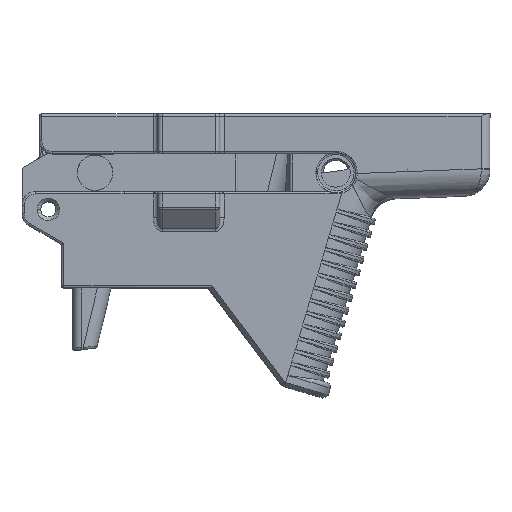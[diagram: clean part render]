
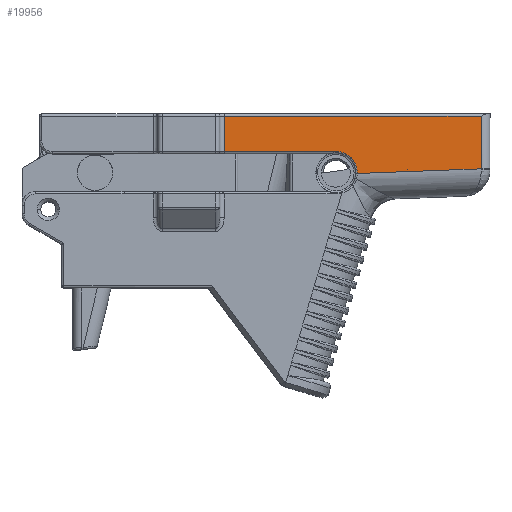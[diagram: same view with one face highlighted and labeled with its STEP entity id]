
A CAD part, top view. The second image highlights one B-rep face of the part: STEP entity #19956.
In plain terms, the highlighted planar face has unit normal (0, 0, 1).
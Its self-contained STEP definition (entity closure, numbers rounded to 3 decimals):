
#33 = LINE ( 'NONE', #19296, #10130 ) ;
#641 = CARTESIAN_POINT ( 'NONE',  ( -48.401, -16.834, 20. ) ) ;
#1420 = CARTESIAN_POINT ( 'NONE',  ( -19.732, -18.269, 20. ) ) ;
#1574 = CARTESIAN_POINT ( 'NONE',  ( -18.826, -19.573, 20. ) ) ;
#1768 = LINE ( 'NONE', #29862, #4794 ) ;
#1918 = EDGE_CURVE ( 'NONE', #3458, #27652, #27993, .T. ) ;
#1987 = VECTOR ( 'NONE', #25201, 1000. ) ;
#2001 = DIRECTION ( 'NONE',  ( 1., 0., 0. ) ) ;
#2130 = CARTESIAN_POINT ( 'NONE',  ( -22.304, -16.888, 20. ) ) ;
#2951 = LINE ( 'NONE', #641, #16053 ) ;
#3097 = CARTESIAN_POINT ( 'NONE',  ( -19.732, -18.269, 20. ) ) ;
#3452 = CARTESIAN_POINT ( 'NONE',  ( -7.079, -20.83, 20. ) ) ;
#3458 = VERTEX_POINT ( 'NONE', #3097 ) ;
#3650 = LINE ( 'NONE', #24642, #8171 ) ;
#3836 = CARTESIAN_POINT ( 'NONE',  ( -22.772, -16.821, 20. ) ) ;
#3881 = CARTESIAN_POINT ( 'NONE',  ( -19.232, -18.88, 20. ) ) ;
#4056 = CARTESIAN_POINT ( 'NONE',  ( -23.365, -16.81, 20. ) ) ;
#4072 = VERTEX_POINT ( 'NONE', #4056 ) ;
#4141 = CARTESIAN_POINT ( 'NONE',  ( -23.167, -16.81, 20. ) ) ;
#4289 = CARTESIAN_POINT ( 'NONE',  ( -21.907, -16.967, 20. ) ) ;
#4794 = VECTOR ( 'NONE', #6690, 1000. ) ;
#4997 = EDGE_CURVE ( 'NONE', #20384, #25131, #26911, .T. ) ;
#5338 = LINE ( 'NONE', #9688, #8516 ) ;
#5424 = EDGE_CURVE ( 'NONE', #12970, #10039, #16466, .T. ) ;
#5905 = CARTESIAN_POINT ( 'NONE',  ( -19.622, -18.383, 20. ) ) ;
#5996 = DIRECTION ( 'NONE',  ( 0., 0., 1. ) ) ;
#6203 = CARTESIAN_POINT ( 'NONE',  ( -19.324, -18.751, 20. ) ) ;
#6354 = CARTESIAN_POINT ( 'NONE',  ( -18.485, -20.649, 20. ) ) ;
#6442 = VECTOR ( 'NONE', #19225, 1000. ) ;
#6464 = CARTESIAN_POINT ( 'NONE',  ( -22.537, -16.851, 20. ) ) ;
#6690 = DIRECTION ( 'NONE',  ( -0.999, -0.037, 0. ) ) ;
#7257 = ORIENTED_EDGE ( 'NONE', *, *, #5424, .F. ) ;
#8138 = DIRECTION ( 'NONE',  ( 0., -1., 0. ) ) ;
#8170 = LINE ( 'NONE', #14798, #9673 ) ;
#8171 = VECTOR ( 'NONE', #8138, 1000. ) ;
#8516 = VECTOR ( 'NONE', #19075, 1000. ) ;
#8923 = B_SPLINE_CURVE_WITH_KNOTS ( 'NONE', 3,
 ( #4141, #22808, #3836, #6464, #16027, #2130, #4289, #20498, #23257, #23104, #25134, #11248, #22955, #27618, #9090, #25284 ),
 .UNSPECIFIED., .F., .F.,
 ( 4, 1, 2, 2, 2, 1, 2, 2, 4 ),
 ( 0., 0.063, 0.094, 0.125, 0.25, 0.313, 0.344, 0.375, 0.5 ),
 .UNSPECIFIED. ) ;
#9090 = CARTESIAN_POINT ( 'NONE',  ( -19.952, -18.041, 20. ) ) ;
#9254 = CARTESIAN_POINT ( 'NONE',  ( -76.723, -16.81, 20. ) ) ;
#9367 = CARTESIAN_POINT ( 'NONE',  ( -48.401, -8.822, 20. ) ) ;
#9673 = VECTOR ( 'NONE', #17415, 1000. ) ;
#9688 = CARTESIAN_POINT ( 'NONE',  ( 9.532, -32.155, 20. ) ) ;
#10039 = VERTEX_POINT ( 'NONE', #11612 ) ;
#10130 = VECTOR ( 'NONE', #19145, 1000. ) ;
#10252 = ORIENTED_EDGE ( 'NONE', *, *, #11085, .F. ) ;
#10475 = PLANE ( 'NONE',  #20900 ) ;
#10712 = VERTEX_POINT ( 'NONE', #14435 ) ;
#10947 = CARTESIAN_POINT ( 'NONE',  ( -18.397, -21.754, 20. ) ) ;
#11039 = VECTOR ( 'NONE', #2001, 1000. ) ;
#11085 = EDGE_CURVE ( 'NONE', #12878, #27652, #1768, .T. ) ;
#11136 = CARTESIAN_POINT ( 'NONE',  ( -18.386, -21.436, 20. ) ) ;
#11248 = CARTESIAN_POINT ( 'NONE',  ( -20.589, -17.565, 20. ) ) ;
#11612 = CARTESIAN_POINT ( 'NONE',  ( 9.532, -8.822, 20. ) ) ;
#12792 = FACE_BOUND ( 'NONE', #21807, .T. ) ;
#12878 = VERTEX_POINT ( 'NONE', #26046 ) ;
#12970 = VERTEX_POINT ( 'NONE', #9367 ) ;
#13366 = CARTESIAN_POINT ( 'NONE',  ( -7.079, -20.83, 20. ) ) ;
#13538 = CARTESIAN_POINT ( 'NONE',  ( -48.401, -16.834, 20. ) ) ;
#13646 = ORIENTED_EDGE ( 'NONE', *, *, #19708, .T. ) ;
#13725 = LINE ( 'NONE', #9254, #11039 ) ;
#14435 = CARTESIAN_POINT ( 'NONE',  ( -7.085, -20.827, 20. ) ) ;
#14798 = CARTESIAN_POINT ( 'NONE',  ( -7.085, -20.827, 20. ) ) ;
#15626 = CARTESIAN_POINT ( 'NONE',  ( -19.189, -18.944, 20. ) ) ;
#15772 = CARTESIAN_POINT ( 'NONE',  ( -18.47, -20.73, 20. ) ) ;
#16027 = CARTESIAN_POINT ( 'NONE',  ( -22.38, -16.874, 20. ) ) ;
#16053 = VECTOR ( 'NONE', #28879, 1000. ) ;
#16466 = LINE ( 'NONE', #16620, #6442 ) ;
#16620 = CARTESIAN_POINT ( 'NONE',  ( -60.491, -8.822, 20. ) ) ;
#16989 = EDGE_CURVE ( 'NONE', #10039, #12878, #5338, .T. ) ;
#17415 = DIRECTION ( 'NONE',  ( 0.866, -0.5, 0. ) ) ;
#17580 = EDGE_LOOP ( 'NONE', ( #29816, #7257, #20981, #19846, #13646, #25649, #26969, #10252 ) ) ;
#17833 = ORIENTED_EDGE ( 'NONE', *, *, #4997, .T. ) ;
#18070 = CARTESIAN_POINT ( 'NONE',  ( -18.52, -20.491, 20. ) ) ;
#19075 = DIRECTION ( 'NONE',  ( 0., -1., 0. ) ) ;
#19145 = DIRECTION ( 'NONE',  ( 0.866, 0.5, 0. ) ) ;
#19225 = DIRECTION ( 'NONE',  ( 1., 0., 0. ) ) ;
#19296 = CARTESIAN_POINT ( 'NONE',  ( -7.091, -20.831, 20. ) ) ;
#19708 = EDGE_CURVE ( 'NONE', #4072, #28724, #13725, .T. ) ;
#19846 = ORIENTED_EDGE ( 'NONE', *, *, #21793, .T. ) ;
#19956 = ADVANCED_FACE ( 'NONE', ( #12792, #22182 ), #10475, .T. ) ;
#20384 = VERTEX_POINT ( 'NONE', #13366 ) ;
#20498 = CARTESIAN_POINT ( 'NONE',  ( -21.599, -17.063, 20. ) ) ;
#20538 = CARTESIAN_POINT ( 'NONE',  ( -18.397, -21.754, 20. ) ) ;
#20900 = AXIS2_PLACEMENT_3D ( 'NONE', #29299, #5996, #24811 ) ;
#20981 = ORIENTED_EDGE ( 'NONE', *, *, #22186, .T. ) ;
#21563 = ORIENTED_EDGE ( 'NONE', *, *, #27503, .T. ) ;
#21613 = EDGE_CURVE ( 'NONE', #25131, #10712, #33, .T. ) ;
#21793 = EDGE_CURVE ( 'NONE', #28483, #4072, #2951, .T. ) ;
#21807 = EDGE_LOOP ( 'NONE', ( #22291, #21563, #17833 ) ) ;
#22182 = FACE_OUTER_BOUND ( 'NONE', #17580, .T. ) ;
#22186 = EDGE_CURVE ( 'NONE', #12970, #28483, #3650, .T. ) ;
#22291 = ORIENTED_EDGE ( 'NONE', *, *, #21613, .T. ) ;
#22702 = CARTESIAN_POINT ( 'NONE',  ( -18.971, -19.285, 20. ) ) ;
#22808 = CARTESIAN_POINT ( 'NONE',  ( -23.009, -16.81, 20. ) ) ;
#22850 = CARTESIAN_POINT ( 'NONE',  ( -18.406, -21.121, 20. ) ) ;
#22955 = CARTESIAN_POINT ( 'NONE',  ( -20.519, -17.611, 20. ) ) ;
#23104 = CARTESIAN_POINT ( 'NONE',  ( -20.935, -17.358, 20. ) ) ;
#23257 = CARTESIAN_POINT ( 'NONE',  ( -21.152, -17.253, 20. ) ) ;
#23948 = CARTESIAN_POINT ( 'NONE',  ( -23.167, -16.81, 20. ) ) ;
#24642 = CARTESIAN_POINT ( 'NONE',  ( -48.401, -12.847, 20. ) ) ;
#24774 = CARTESIAN_POINT ( 'NONE',  ( -7.091, -20.831, 20. ) ) ;
#24811 = DIRECTION ( 'NONE',  ( 1., 0., 0. ) ) ;
#25032 = CARTESIAN_POINT ( 'NONE',  ( -18.652, -20.026, 20. ) ) ;
#25131 = VERTEX_POINT ( 'NONE', #24774 ) ;
#25134 = CARTESIAN_POINT ( 'NONE',  ( -20.726, -17.48, 20. ) ) ;
#25201 = DIRECTION ( 'NONE',  ( -0.999, -0.037, 0. ) ) ;
#25284 = CARTESIAN_POINT ( 'NONE',  ( -19.732, -18.269, 20. ) ) ;
#25649 = ORIENTED_EDGE ( 'NONE', *, *, #27581, .T. ) ;
#26046 = CARTESIAN_POINT ( 'NONE',  ( 9.532, -20.71, 20. ) ) ;
#26911 = LINE ( 'NONE', #3452, #1987 ) ;
#26969 = ORIENTED_EDGE ( 'NONE', *, *, #1918, .T. ) ;
#27352 = CARTESIAN_POINT ( 'NONE',  ( -19.466, -18.561, 20. ) ) ;
#27503 = EDGE_CURVE ( 'NONE', #10712, #20384, #8170, .T. ) ;
#27581 = EDGE_CURVE ( 'NONE', #28724, #3458, #8923, .T. ) ;
#27618 = CARTESIAN_POINT ( 'NONE',  ( -20.193, -17.836, 20. ) ) ;
#27652 = VERTEX_POINT ( 'NONE', #10947 ) ;
#27993 = B_SPLINE_CURVE_WITH_KNOTS ( 'NONE', 3,
 ( #1420, #5905, #27352, #6203, #3881, #15626, #22702, #1574, #25032, #29817, #18070, #6354, #15772, #22850, #11136, #20538 ),
 .UNSPECIFIED., .F., .F.,
 ( 4, 1, 2, 2, 2, 1, 2, 2, 4 ),
 ( 0.5, 0.563, 0.594, 0.625, 0.75, 0.813, 0.844, 0.875, 1. ),
 .UNSPECIFIED. ) ;
#28483 = VERTEX_POINT ( 'NONE', #13538 ) ;
#28724 = VERTEX_POINT ( 'NONE', #23948 ) ;
#28879 = DIRECTION ( 'NONE',  ( 1., 0.001, 0. ) ) ;
#29299 = CARTESIAN_POINT ( 'NONE',  ( -76.723, -12.847, 20. ) ) ;
#29816 = ORIENTED_EDGE ( 'NONE', *, *, #16989, .F. ) ;
#29817 = CARTESIAN_POINT ( 'NONE',  ( -18.577, -20.256, 20. ) ) ;
#29862 = CARTESIAN_POINT ( 'NONE',  ( -19.877, -21.809, 20. ) ) ;
